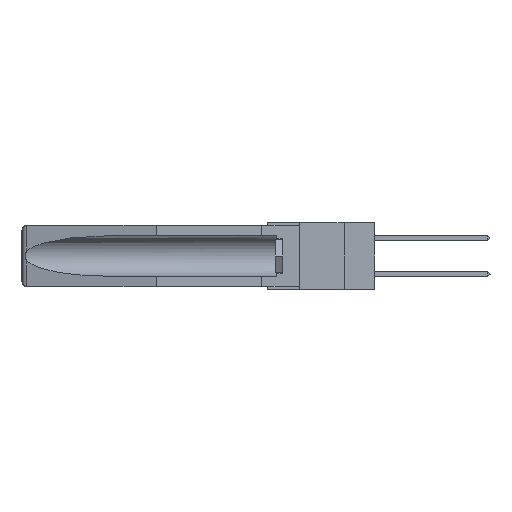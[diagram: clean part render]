
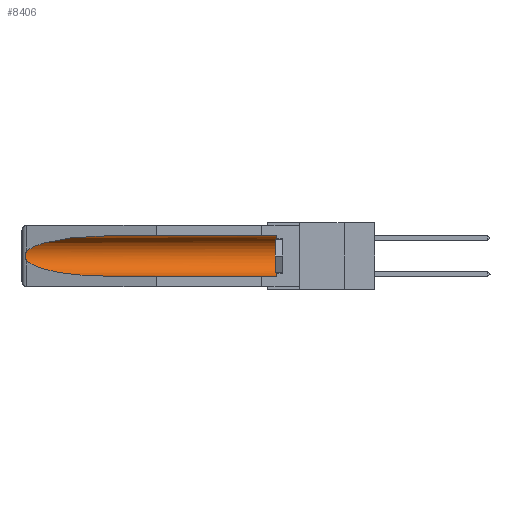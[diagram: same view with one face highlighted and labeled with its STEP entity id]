
A CAD part, left-side view. The second image highlights one B-rep face of the part: STEP entity #8406.
In plain terms, the highlighted cylindrical face has radius 2.857 mm (diameter 5.715 mm), a partial arc.
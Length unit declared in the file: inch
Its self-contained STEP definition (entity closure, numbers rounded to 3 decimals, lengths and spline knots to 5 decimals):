
#756 = ORIENTED_EDGE ( 'NONE', *, *, #3388, .T. ) ;
#868 = CARTESIAN_POINT ( 'NONE',  ( 0.26537, 1.52718, -0.14972 ) ) ;
#1080 = CARTESIAN_POINT ( 'NONE',  ( 0.2673, 1.53269, -0.17917 ) ) ;
#1149 = VECTOR ( 'NONE', #18209, 39.37008 ) ;
#1260 = EDGE_CURVE ( 'NONE', #8086, #4215, #4276, .T. ) ;
#1480 = CARTESIAN_POINT ( 'NONE',  ( 0.26537, 1.52718, -0.19328 ) ) ;
#2356 = DIRECTION ( 'NONE',  ( 0., 1., 0. ) ) ;
#2729 = CARTESIAN_POINT ( 'NONE',  ( 0.26537, 1.52718, -0.19328 ) ) ;
#2742 = CARTESIAN_POINT ( 'NONE',  ( 0.26654, 1.53092, -0.15636 ) ) ;
#2805 = CARTESIAN_POINT ( 'NONE',  ( 0.26655, 1.53094, -0.18657 ) ) ;
#3388 = EDGE_CURVE ( 'NONE', #11662, #17155, #17562, .T. ) ;
#3664 =( BOUNDED_CURVE ( )  B_SPLINE_CURVE ( 3, ( #5454, #10128, #16277, #868 ),
 .UNSPECIFIED., .F., .T. ) 
 B_SPLINE_CURVE_WITH_KNOTS ( ( 4, 4 ),
 ( 4.71239, 6.08839 ),
 .UNSPECIFIED. ) 
 CURVE ( )  GEOMETRIC_REPRESENTATION_ITEM ( )  RATIONAL_B_SPLINE_CURVE ( ( 1., 0.848, 0.848, 1. ) ) 
 REPRESENTATION_ITEM ( '' )  );
#3814 = EDGE_CURVE ( 'NONE', #4958, #4215, #18988, .T. ) ;
#4198 = CARTESIAN_POINT ( 'NONE',  ( 0.2675, 1.53308, -0.17534 ) ) ;
#4215 = VERTEX_POINT ( 'NONE', #15493 ) ;
#4276 =( BOUNDED_CURVE ( )  B_SPLINE_CURVE ( 3, ( #1480, #10658, #18093, #12461 ),
 .UNSPECIFIED., .F., .F. ) 
 B_SPLINE_CURVE_WITH_KNOTS ( ( 4, 4 ),
 ( 0.1948, 1.5708 ),
 .UNSPECIFIED. ) 
 CURVE ( )  GEOMETRIC_REPRESENTATION_ITEM ( )  RATIONAL_B_SPLINE_CURVE ( ( 1., 0.848, 0.848, 1. ) ) 
 REPRESENTATION_ITEM ( '' )  );
#4475 = AXIS2_PLACEMENT_3D ( 'NONE', #9662, #15695, #6683 ) ;
#4958 = VERTEX_POINT ( 'NONE', #17953 ) ;
#5359 = FACE_OUTER_BOUND ( 'NONE', #15186, .T. ) ;
#5454 = CARTESIAN_POINT ( 'NONE',  ( 0.155, 1.07973, -0.059 ) ) ;
#5730 = CARTESIAN_POINT ( 'NONE',  ( 0.2673, 1.5327, -0.16383 ) ) ;
#6425 = CARTESIAN_POINT ( 'NONE',  ( 0.155, -0.30754, -0.059 ) ) ;
#6683 = DIRECTION ( 'NONE',  ( 0., 0., 1. ) ) ;
#6844 = ORIENTED_EDGE ( 'NONE', *, *, #12689, .T. ) ;
#7000 = AXIS2_PLACEMENT_3D ( 'NONE', #11454, #2356, #15842 ) ;
#7815 = ORIENTED_EDGE ( 'NONE', *, *, #3814, .F. ) ;
#8086 = VERTEX_POINT ( 'NONE', #2729 ) ;
#8406 = ADVANCED_FACE ( 'NONE', ( #5359 ), #10611, .F. ) ;
#8429 = CARTESIAN_POINT ( 'NONE',  ( 0.155, 0.126, -0.059 ) ) ;
#9662 = CARTESIAN_POINT ( 'NONE',  ( 0.155, 0.126, -0.1715 ) ) ;
#10128 = CARTESIAN_POINT ( 'NONE',  ( 0.21114, 1.30732, -0.059 ) ) ;
#10266 = CARTESIAN_POINT ( 'NONE',  ( 0.26537, 1.52718, -0.19328 ) ) ;
#10450 = CARTESIAN_POINT ( 'NONE',  ( 0.155, -0.30754, -0.284 ) ) ;
#10536 = EDGE_CURVE ( 'NONE', #19453, #8086, #11326, .T. ) ;
#10611 = CYLINDRICAL_SURFACE ( 'NONE', #7000, 0.1125 ) ;
#10658 = CARTESIAN_POINT ( 'NONE',  ( 0.25451, 1.48313, -0.24835 ) ) ;
#11197 = DIRECTION ( 'NONE',  ( 0., 1., 0. ) ) ;
#11238 = ORIENTED_EDGE ( 'NONE', *, *, #10536, .T. ) ;
#11326 = B_SPLINE_CURVE_WITH_KNOTS ( 'NONE', 3,
 ( #19553, #16286, #2742, #5730, #11908, #4198, #1080, #2805, #16352, #10266 ),
 .UNSPECIFIED., .F., .F.,
 ( 4, 2, 2, 2, 4 ),
 ( 0., 0.00029, 0.00058, 0.00087, 0.00117 ),
 .UNSPECIFIED. ) ;
#11454 = CARTESIAN_POINT ( 'NONE',  ( 0.155, -0.30754, -0.1715 ) ) ;
#11497 = CIRCLE ( 'NONE', #4475, 0.1125 ) ;
#11662 = VERTEX_POINT ( 'NONE', #8429 ) ;
#11908 = CARTESIAN_POINT ( 'NONE',  ( 0.2675, 1.53308, -0.16763 ) ) ;
#12060 = ORIENTED_EDGE ( 'NONE', *, *, #1260, .T. ) ;
#12461 = CARTESIAN_POINT ( 'NONE',  ( 0.155, 1.07973, -0.284 ) ) ;
#12689 = EDGE_CURVE ( 'NONE', #4958, #11662, #11497, .T. ) ;
#12893 = EDGE_CURVE ( 'NONE', #17155, #19453, #3664, .T. ) ;
#15175 = ORIENTED_EDGE ( 'NONE', *, *, #12893, .T. ) ;
#15186 = EDGE_LOOP ( 'NONE', ( #15175, #11238, #12060, #7815, #6844, #756 ) ) ;
#15493 = CARTESIAN_POINT ( 'NONE',  ( 0.155, 1.07973, -0.284 ) ) ;
#15695 = DIRECTION ( 'NONE',  ( 0., -1., 0. ) ) ;
#15842 = DIRECTION ( 'NONE',  ( 0., 0., 1. ) ) ;
#16277 = CARTESIAN_POINT ( 'NONE',  ( 0.25451, 1.48313, -0.09465 ) ) ;
#16286 = CARTESIAN_POINT ( 'NONE',  ( 0.26597, 1.52961, -0.15275 ) ) ;
#16352 = CARTESIAN_POINT ( 'NONE',  ( 0.26597, 1.5296, -0.19026 ) ) ;
#17155 = VERTEX_POINT ( 'NONE', #19265 ) ;
#17328 = VECTOR ( 'NONE', #11197, 39.37008 ) ;
#17562 = LINE ( 'NONE', #6425, #17328 ) ;
#17953 = CARTESIAN_POINT ( 'NONE',  ( 0.155, 0.126, -0.284 ) ) ;
#18093 = CARTESIAN_POINT ( 'NONE',  ( 0.21114, 1.30732, -0.284 ) ) ;
#18209 = DIRECTION ( 'NONE',  ( 0., 1., 0. ) ) ;
#18313 = CARTESIAN_POINT ( 'NONE',  ( 0.26537, 1.52718, -0.14972 ) ) ;
#18988 = LINE ( 'NONE', #10450, #1149 ) ;
#19265 = CARTESIAN_POINT ( 'NONE',  ( 0.155, 1.07973, -0.059 ) ) ;
#19453 = VERTEX_POINT ( 'NONE', #18313 ) ;
#19553 = CARTESIAN_POINT ( 'NONE',  ( 0.26537, 1.52718, -0.14972 ) ) ;
